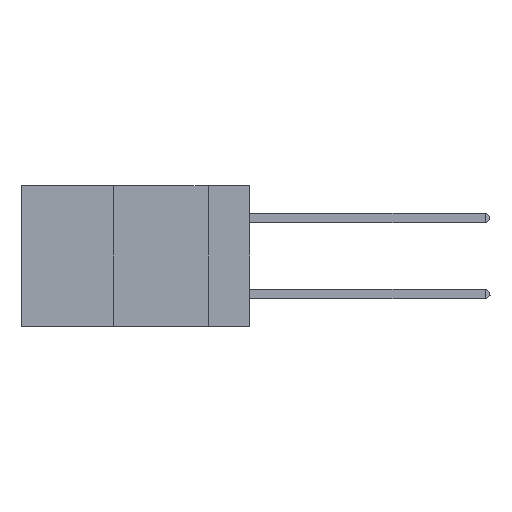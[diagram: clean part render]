
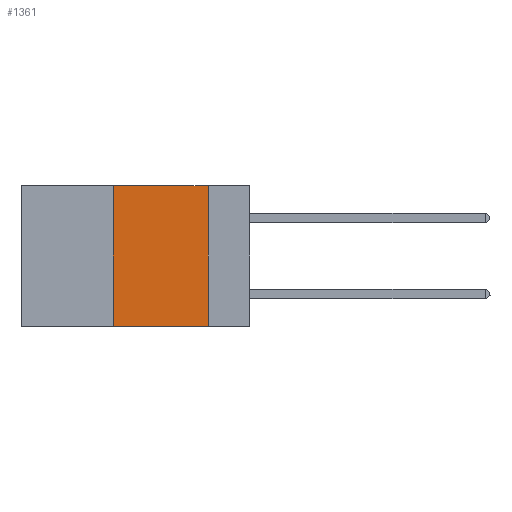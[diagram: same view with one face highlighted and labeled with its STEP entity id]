
A CAD part, left-side view. The second image highlights one B-rep face of the part: STEP entity #1361.
In plain terms, the highlighted planar face has unit normal (-1, 0, 0).
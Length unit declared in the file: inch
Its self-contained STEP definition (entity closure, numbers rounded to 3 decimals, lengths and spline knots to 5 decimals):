
#609 = VERTEX_POINT ( 'NONE', #5250 ) ;
#1361 = ADVANCED_FACE ( 'NONE', ( #3328 ), #21110, .F. ) ;
#1751 = VECTOR ( 'NONE', #7676, 39.37008 ) ;
#2515 = CARTESIAN_POINT ( 'NONE',  ( 0., 0.11, 0. ) ) ;
#2630 = CARTESIAN_POINT ( 'NONE',  ( 0., 0.36, 0. ) ) ;
#3141 = VECTOR ( 'NONE', #14576, 39.37008 ) ;
#3328 = FACE_OUTER_BOUND ( 'NONE', #9607, .T. ) ;
#3382 = CARTESIAN_POINT ( 'NONE',  ( 0., 0.6, -0.37 ) ) ;
#3952 = ORIENTED_EDGE ( 'NONE', *, *, #10053, .F. ) ;
#3955 = DIRECTION ( 'NONE',  ( 1., 0., 0. ) ) ;
#4443 = CARTESIAN_POINT ( 'NONE',  ( 0., 0.6, 0. ) ) ;
#4770 = ORIENTED_EDGE ( 'NONE', *, *, #13210, .F. ) ;
#5250 = CARTESIAN_POINT ( 'NONE',  ( 0., 0.11, -0.37 ) ) ;
#5278 = VECTOR ( 'NONE', #8292, 39.37008 ) ;
#5814 = ORIENTED_EDGE ( 'NONE', *, *, #8922, .T. ) ;
#6675 = VERTEX_POINT ( 'NONE', #2630 ) ;
#7148 = LINE ( 'NONE', #16039, #1751 ) ;
#7676 = DIRECTION ( 'NONE',  ( 0., 0., -1. ) ) ;
#7996 = LINE ( 'NONE', #8947, #18554 ) ;
#8292 = DIRECTION ( 'NONE',  ( 0., -1., 0. ) ) ;
#8324 = VERTEX_POINT ( 'NONE', #20241 ) ;
#8922 = EDGE_CURVE ( 'NONE', #8324, #609, #9653, .T. ) ;
#8947 = CARTESIAN_POINT ( 'NONE',  ( 0., 0.36, 0. ) ) ;
#9223 = VERTEX_POINT ( 'NONE', #2515 ) ;
#9241 = CARTESIAN_POINT ( 'NONE',  ( 0., 0.6, 0. ) ) ;
#9607 = EDGE_LOOP ( 'NONE', ( #4770, #3952, #12034, #5814 ) ) ;
#9653 = LINE ( 'NONE', #3382, #5278 ) ;
#10053 = EDGE_CURVE ( 'NONE', #6675, #9223, #19913, .T. ) ;
#11389 = AXIS2_PLACEMENT_3D ( 'NONE', #4443, #3955, #14204 ) ;
#12034 = ORIENTED_EDGE ( 'NONE', *, *, #12447, .F. ) ;
#12280 = DIRECTION ( 'NONE',  ( 0., 0., 1. ) ) ;
#12447 = EDGE_CURVE ( 'NONE', #8324, #6675, #7996, .T. ) ;
#13210 = EDGE_CURVE ( 'NONE', #9223, #609, #7148, .T. ) ;
#14204 = DIRECTION ( 'NONE',  ( 0., 0., -1. ) ) ;
#14576 = DIRECTION ( 'NONE',  ( 0., -1., 0. ) ) ;
#16039 = CARTESIAN_POINT ( 'NONE',  ( 0., 0.11, 0. ) ) ;
#18554 = VECTOR ( 'NONE', #12280, 39.37008 ) ;
#19913 = LINE ( 'NONE', #9241, #3141 ) ;
#20241 = CARTESIAN_POINT ( 'NONE',  ( 0., 0.36, -0.37 ) ) ;
#21110 = PLANE ( 'NONE',  #11389 ) ;
